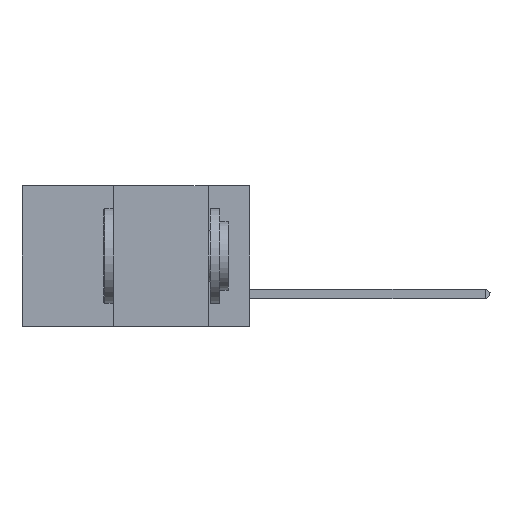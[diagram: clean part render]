
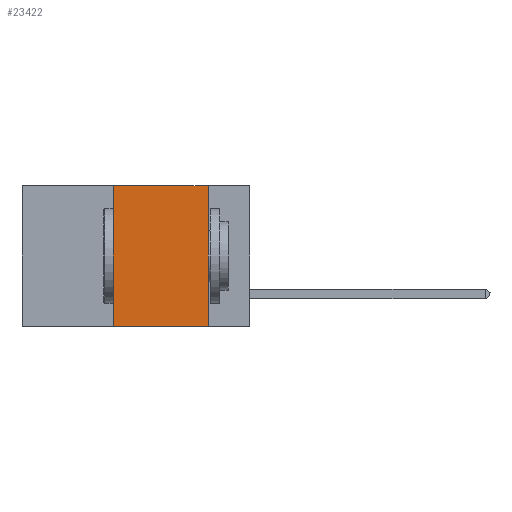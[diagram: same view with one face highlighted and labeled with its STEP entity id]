
A CAD part, left-side view. The second image highlights one B-rep face of the part: STEP entity #23422.
In plain terms, the highlighted planar face has unit normal (-1, 0, 0).
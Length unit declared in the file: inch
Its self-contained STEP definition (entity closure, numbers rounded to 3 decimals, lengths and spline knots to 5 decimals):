
#161 = VECTOR ( 'NONE', #10357, 39.37008 ) ;
#349 = LINE ( 'NONE', #9078, #12222 ) ;
#491 = LINE ( 'NONE', #704, #161 ) ;
#628 = CARTESIAN_POINT ( 'NONE',  ( 0., 0.11, -0.37 ) ) ;
#704 = CARTESIAN_POINT ( 'NONE',  ( 0., 0.11, 0. ) ) ;
#1499 = AXIS2_PLACEMENT_3D ( 'NONE', #6535, #4244, #22691 ) ;
#1953 = CARTESIAN_POINT ( 'NONE',  ( 0., 0.36, 0. ) ) ;
#2532 = ORIENTED_EDGE ( 'NONE', *, *, #23768, .F. ) ;
#4244 = DIRECTION ( 'NONE',  ( 1., 0., 0. ) ) ;
#6535 = CARTESIAN_POINT ( 'NONE',  ( 0., 0.6, 0. ) ) ;
#6910 = FACE_OUTER_BOUND ( 'NONE', #15900, .T. ) ;
#9078 = CARTESIAN_POINT ( 'NONE',  ( 0., 0.6, 0. ) ) ;
#10357 = DIRECTION ( 'NONE',  ( 0., 0., -1. ) ) ;
#11176 = VECTOR ( 'NONE', #11514, 39.37008 ) ;
#11189 = PLANE ( 'NONE',  #1499 ) ;
#11320 = EDGE_CURVE ( 'NONE', #19074, #26680, #349, .T. ) ;
#11339 = DIRECTION ( 'NONE',  ( 0., -1., 0. ) ) ;
#11514 = DIRECTION ( 'NONE',  ( 0., 0., 1. ) ) ;
#12222 = VECTOR ( 'NONE', #11339, 39.37008 ) ;
#13019 = LINE ( 'NONE', #1953, #11176 ) ;
#14838 = LINE ( 'NONE', #22381, #17391 ) ;
#15692 = ORIENTED_EDGE ( 'NONE', *, *, #11320, .F. ) ;
#15900 = EDGE_LOOP ( 'NONE', ( #2532, #15692, #22497, #16064 ) ) ;
#16064 = ORIENTED_EDGE ( 'NONE', *, *, #16940, .T. ) ;
#16720 = EDGE_CURVE ( 'NONE', #17977, #19074, #13019, .T. ) ;
#16940 = EDGE_CURVE ( 'NONE', #17977, #22636, #14838, .T. ) ;
#17391 = VECTOR ( 'NONE', #29207, 39.37008 ) ;
#17977 = VERTEX_POINT ( 'NONE', #26721 ) ;
#19074 = VERTEX_POINT ( 'NONE', #29051 ) ;
#22381 = CARTESIAN_POINT ( 'NONE',  ( 0., 0.6, -0.37 ) ) ;
#22497 = ORIENTED_EDGE ( 'NONE', *, *, #16720, .F. ) ;
#22636 = VERTEX_POINT ( 'NONE', #628 ) ;
#22691 = DIRECTION ( 'NONE',  ( 0., 0., -1. ) ) ;
#23189 = CARTESIAN_POINT ( 'NONE',  ( 0., 0.11, 0. ) ) ;
#23422 = ADVANCED_FACE ( 'NONE', ( #6910 ), #11189, .F. ) ;
#23768 = EDGE_CURVE ( 'NONE', #26680, #22636, #491, .T. ) ;
#26680 = VERTEX_POINT ( 'NONE', #23189 ) ;
#26721 = CARTESIAN_POINT ( 'NONE',  ( 0., 0.36, -0.37 ) ) ;
#29051 = CARTESIAN_POINT ( 'NONE',  ( 0., 0.36, 0. ) ) ;
#29207 = DIRECTION ( 'NONE',  ( 0., -1., 0. ) ) ;
